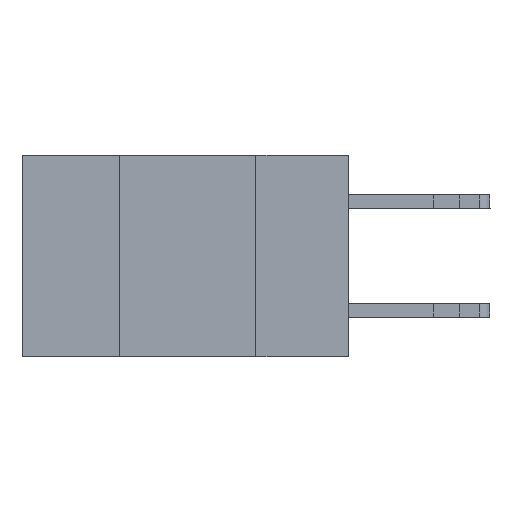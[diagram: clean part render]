
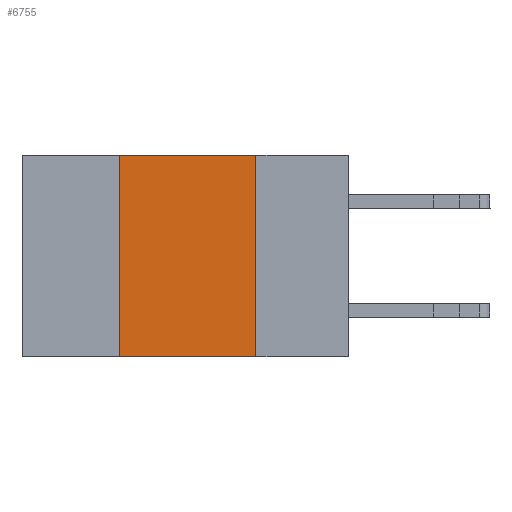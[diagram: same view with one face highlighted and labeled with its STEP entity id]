
A CAD part, left-side view. The second image highlights one B-rep face of the part: STEP entity #6755.
In plain terms, the highlighted planar face has unit normal (-1, 0, 0).
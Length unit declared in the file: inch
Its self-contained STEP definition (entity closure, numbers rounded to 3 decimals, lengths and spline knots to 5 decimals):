
#108 = VERTEX_POINT ( 'NONE', #10538 ) ;
#582 = DIRECTION ( 'NONE',  ( 0., -1., 0. ) ) ;
#1155 = CARTESIAN_POINT ( 'NONE',  ( 0., 0.42, 0. ) ) ;
#1698 = VECTOR ( 'NONE', #582, 39.37008 ) ;
#1949 = VECTOR ( 'NONE', #2863, 39.37008 ) ;
#2863 = DIRECTION ( 'NONE',  ( 0., -1., 0. ) ) ;
#3026 = CARTESIAN_POINT ( 'NONE',  ( 0., 0.6, 0. ) ) ;
#3315 = VERTEX_POINT ( 'NONE', #4484 ) ;
#3796 = VECTOR ( 'NONE', #7205, 39.37008 ) ;
#3799 = AXIS2_PLACEMENT_3D ( 'NONE', #3026, #6772, #13182 ) ;
#4002 = LINE ( 'NONE', #6600, #1698 ) ;
#4484 = CARTESIAN_POINT ( 'NONE',  ( 0., 0.17, -0.37 ) ) ;
#5782 = ORIENTED_EDGE ( 'NONE', *, *, #8467, .F. ) ;
#6430 = CARTESIAN_POINT ( 'NONE',  ( 0., 0.17, 0. ) ) ;
#6600 = CARTESIAN_POINT ( 'NONE',  ( 0., 0.6, 0. ) ) ;
#6755 = ADVANCED_FACE ( 'NONE', ( #11607 ), #8102, .F. ) ;
#6772 = DIRECTION ( 'NONE',  ( 1., 0., 0. ) ) ;
#6790 = EDGE_CURVE ( 'NONE', #108, #3315, #10530, .T. ) ;
#7205 = DIRECTION ( 'NONE',  ( 0., 0., 1. ) ) ;
#8102 = PLANE ( 'NONE',  #3799 ) ;
#8396 = EDGE_LOOP ( 'NONE', ( #14938, #15219, #5782, #11229 ) ) ;
#8467 = EDGE_CURVE ( 'NONE', #108, #11178, #14987, .T. ) ;
#9123 = CARTESIAN_POINT ( 'NONE',  ( 0., 0.6, -0.37 ) ) ;
#10530 = LINE ( 'NONE', #9123, #1949 ) ;
#10538 = CARTESIAN_POINT ( 'NONE',  ( 0., 0.42, -0.37 ) ) ;
#11178 = VERTEX_POINT ( 'NONE', #1155 ) ;
#11229 = ORIENTED_EDGE ( 'NONE', *, *, #6790, .T. ) ;
#11407 = CARTESIAN_POINT ( 'NONE',  ( 0., 0.17, -0.37 ) ) ;
#11486 = DIRECTION ( 'NONE',  ( 0., 0., -1. ) ) ;
#11607 = FACE_OUTER_BOUND ( 'NONE', #8396, .T. ) ;
#12869 = VECTOR ( 'NONE', #11486, 39.37008 ) ;
#13182 = DIRECTION ( 'NONE',  ( 0., 0., -1. ) ) ;
#13633 = CARTESIAN_POINT ( 'NONE',  ( 0., 0.42, -0.37 ) ) ;
#14734 = VERTEX_POINT ( 'NONE', #6430 ) ;
#14864 = EDGE_CURVE ( 'NONE', #11178, #14734, #4002, .T. ) ;
#14938 = ORIENTED_EDGE ( 'NONE', *, *, #15170, .F. ) ;
#14987 = LINE ( 'NONE', #13633, #3796 ) ;
#15170 = EDGE_CURVE ( 'NONE', #14734, #3315, #15185, .T. ) ;
#15185 = LINE ( 'NONE', #11407, #12869 ) ;
#15219 = ORIENTED_EDGE ( 'NONE', *, *, #14864, .F. ) ;
